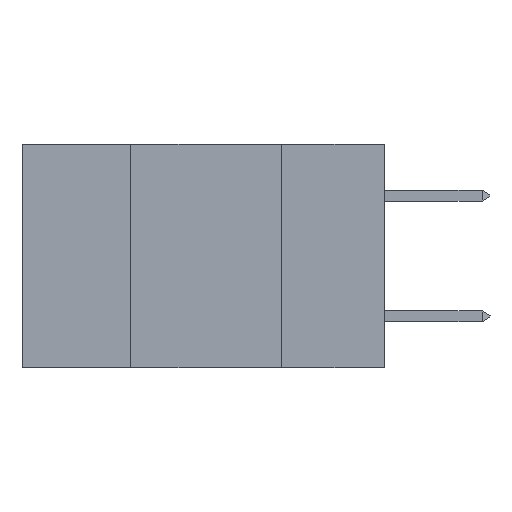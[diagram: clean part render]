
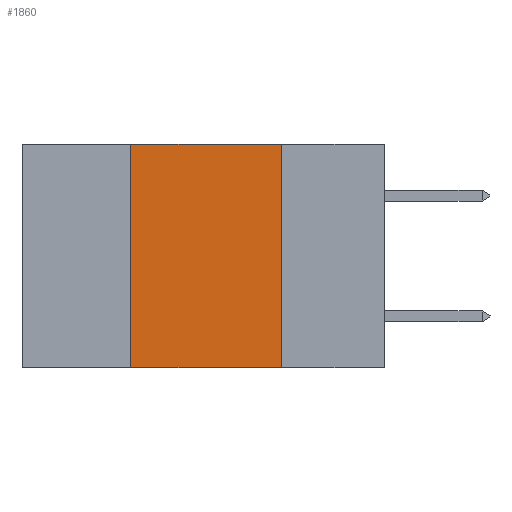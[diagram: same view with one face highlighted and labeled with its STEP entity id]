
A CAD part, left-side view. The second image highlights one B-rep face of the part: STEP entity #1860.
In plain terms, the highlighted planar face has unit normal (-1, 0, 0).
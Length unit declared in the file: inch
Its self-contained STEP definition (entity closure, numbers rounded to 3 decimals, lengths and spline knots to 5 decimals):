
#1 = EDGE_CURVE ( 'NONE', #9244, #943, #22442, .T. ) ;
#388 = CARTESIAN_POINT ( 'NONE',  ( 0., 0.42, -0.37 ) ) ;
#849 = VECTOR ( 'NONE', #9863, 39.37008 ) ;
#943 = VERTEX_POINT ( 'NONE', #16042 ) ;
#1203 = FACE_OUTER_BOUND ( 'NONE', #19218, .T. ) ;
#1860 = ADVANCED_FACE ( 'NONE', ( #1203 ), #3531, .F. ) ;
#3021 = CARTESIAN_POINT ( 'NONE',  ( 0., 0.17, 0. ) ) ;
#3531 = PLANE ( 'NONE',  #21626 ) ;
#4402 = ORIENTED_EDGE ( 'NONE', *, *, #12435, .F. ) ;
#4815 = DIRECTION ( 'NONE',  ( 0., -1., 0. ) ) ;
#6045 = VECTOR ( 'NONE', #20136, 39.37008 ) ;
#6358 = EDGE_CURVE ( 'NONE', #24241, #943, #10422, .T. ) ;
#6896 = CARTESIAN_POINT ( 'NONE',  ( 0., 0.42, 0. ) ) ;
#7049 = ORIENTED_EDGE ( 'NONE', *, *, #1, .F. ) ;
#9244 = VERTEX_POINT ( 'NONE', #15824 ) ;
#9863 = DIRECTION ( 'NONE',  ( 0., 0., 1. ) ) ;
#10422 = LINE ( 'NONE', #21202, #22990 ) ;
#11453 = LINE ( 'NONE', #22077, #25424 ) ;
#12316 = LINE ( 'NONE', #24953, #849 ) ;
#12435 = EDGE_CURVE ( 'NONE', #24241, #26304, #12316, .T. ) ;
#14341 = DIRECTION ( 'NONE',  ( 0., 0., -1. ) ) ;
#15824 = CARTESIAN_POINT ( 'NONE',  ( 0., 0.17, 0. ) ) ;
#16042 = CARTESIAN_POINT ( 'NONE',  ( 0., 0.17, -0.37 ) ) ;
#16626 = DIRECTION ( 'NONE',  ( 1., 0., 0. ) ) ;
#17313 = ORIENTED_EDGE ( 'NONE', *, *, #6358, .T. ) ;
#17705 = ORIENTED_EDGE ( 'NONE', *, *, #27189, .F. ) ;
#19218 = EDGE_LOOP ( 'NONE', ( #7049, #17705, #4402, #17313 ) ) ;
#20136 = DIRECTION ( 'NONE',  ( 0., 0., -1. ) ) ;
#21202 = CARTESIAN_POINT ( 'NONE',  ( 0., 0.6, -0.37 ) ) ;
#21626 = AXIS2_PLACEMENT_3D ( 'NONE', #27683, #16626, #14341 ) ;
#22077 = CARTESIAN_POINT ( 'NONE',  ( 0., 0.6, 0. ) ) ;
#22442 = LINE ( 'NONE', #3021, #6045 ) ;
#22990 = VECTOR ( 'NONE', #27671, 39.37008 ) ;
#24241 = VERTEX_POINT ( 'NONE', #388 ) ;
#24953 = CARTESIAN_POINT ( 'NONE',  ( 0., 0.42, 0. ) ) ;
#25424 = VECTOR ( 'NONE', #4815, 39.37008 ) ;
#26304 = VERTEX_POINT ( 'NONE', #6896 ) ;
#27189 = EDGE_CURVE ( 'NONE', #26304, #9244, #11453, .T. ) ;
#27671 = DIRECTION ( 'NONE',  ( 0., -1., 0. ) ) ;
#27683 = CARTESIAN_POINT ( 'NONE',  ( 0., 0.6, 0. ) ) ;
